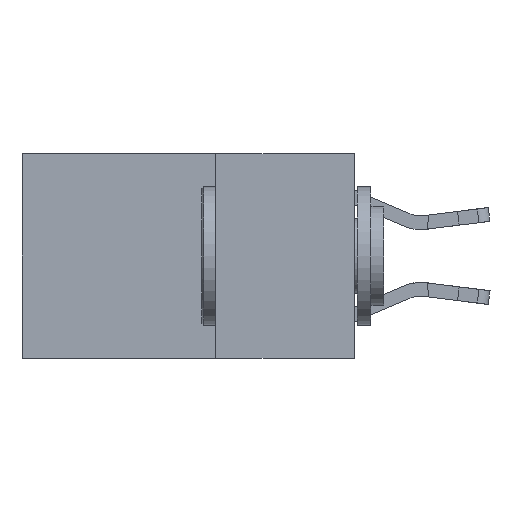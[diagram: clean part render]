
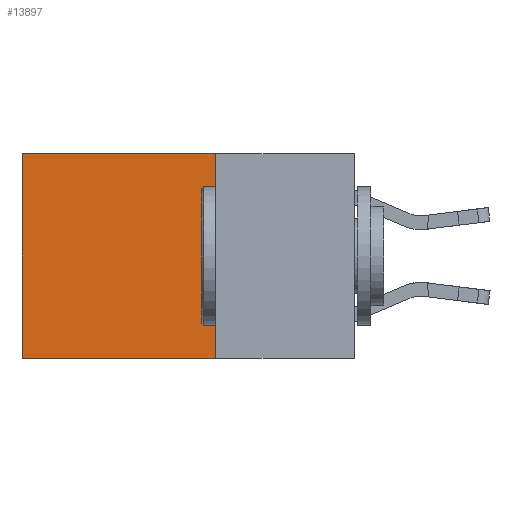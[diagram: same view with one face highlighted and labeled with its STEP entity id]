
A CAD part, left-side view. The second image highlights one B-rep face of the part: STEP entity #13897.
In plain terms, the highlighted planar face has unit normal (-1, 0, 0).
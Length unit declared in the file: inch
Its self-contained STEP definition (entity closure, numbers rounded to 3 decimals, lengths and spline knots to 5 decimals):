
#1834 = ORIENTED_EDGE ( 'NONE', *, *, #20337, .F. ) ;
#2827 = LINE ( 'NONE', #18299, #13389 ) ;
#4273 = AXIS2_PLACEMENT_3D ( 'NONE', #9148, #11145, #24691 ) ;
#5024 = LINE ( 'NONE', #13035, #23940 ) ;
#6374 = DIRECTION ( 'NONE',  ( 0., 1., 0. ) ) ;
#7179 = PLANE ( 'NONE',  #4273 ) ;
#9148 = CARTESIAN_POINT ( 'NONE',  ( 0.2625, 0.25, 0. ) ) ;
#9386 = DIRECTION ( 'NONE',  ( 0., 0., -1. ) ) ;
#11145 = DIRECTION ( 'NONE',  ( 1., 0., 0. ) ) ;
#11464 = EDGE_CURVE ( 'NONE', #17145, #24855, #20064, .T. ) ;
#11680 = EDGE_CURVE ( 'NONE', #22205, #17145, #18240, .T. ) ;
#12310 = DIRECTION ( 'NONE',  ( 0., 1., 0. ) ) ;
#12886 = FACE_OUTER_BOUND ( 'NONE', #23180, .T. ) ;
#13035 = CARTESIAN_POINT ( 'NONE',  ( 0.2625, 0.25, 0. ) ) ;
#13151 = ORIENTED_EDGE ( 'NONE', *, *, #11464, .T. ) ;
#13389 = VECTOR ( 'NONE', #12310, 39.37008 ) ;
#13897 = ADVANCED_FACE ( 'NONE', ( #12886 ), #7179, .F. ) ;
#14247 = VECTOR ( 'NONE', #9386, 39.37008 ) ;
#14612 = EDGE_CURVE ( 'NONE', #22205, #14678, #5024, .T. ) ;
#14650 = ORIENTED_EDGE ( 'NONE', *, *, #14612, .F. ) ;
#14678 = VERTEX_POINT ( 'NONE', #17282 ) ;
#15085 = CARTESIAN_POINT ( 'NONE',  ( 0.2625, 0.25, 0. ) ) ;
#17145 = VERTEX_POINT ( 'NONE', #19496 ) ;
#17282 = CARTESIAN_POINT ( 'NONE',  ( 0.2625, 0.25, -0.37 ) ) ;
#17906 = ORIENTED_EDGE ( 'NONE', *, *, #11680, .T. ) ;
#18240 = LINE ( 'NONE', #20062, #24750 ) ;
#18299 = CARTESIAN_POINT ( 'NONE',  ( 0.2625, 0.25, -0.37 ) ) ;
#19230 = CARTESIAN_POINT ( 'NONE',  ( 0.2625, 0.6, 0. ) ) ;
#19496 = CARTESIAN_POINT ( 'NONE',  ( 0.2625, 0.6, 0. ) ) ;
#20062 = CARTESIAN_POINT ( 'NONE',  ( 0.2625, 0.25, 0. ) ) ;
#20064 = LINE ( 'NONE', #19230, #14247 ) ;
#20337 = EDGE_CURVE ( 'NONE', #14678, #24855, #2827, .T. ) ;
#22205 = VERTEX_POINT ( 'NONE', #15085 ) ;
#23180 = EDGE_LOOP ( 'NONE', ( #13151, #1834, #14650, #17906 ) ) ;
#23940 = VECTOR ( 'NONE', #24660, 39.37008 ) ;
#24660 = DIRECTION ( 'NONE',  ( 0., 0., -1. ) ) ;
#24691 = DIRECTION ( 'NONE',  ( 0., 0., -1. ) ) ;
#24750 = VECTOR ( 'NONE', #6374, 39.37008 ) ;
#24855 = VERTEX_POINT ( 'NONE', #24914 ) ;
#24914 = CARTESIAN_POINT ( 'NONE',  ( 0.2625, 0.6, -0.37 ) ) ;
